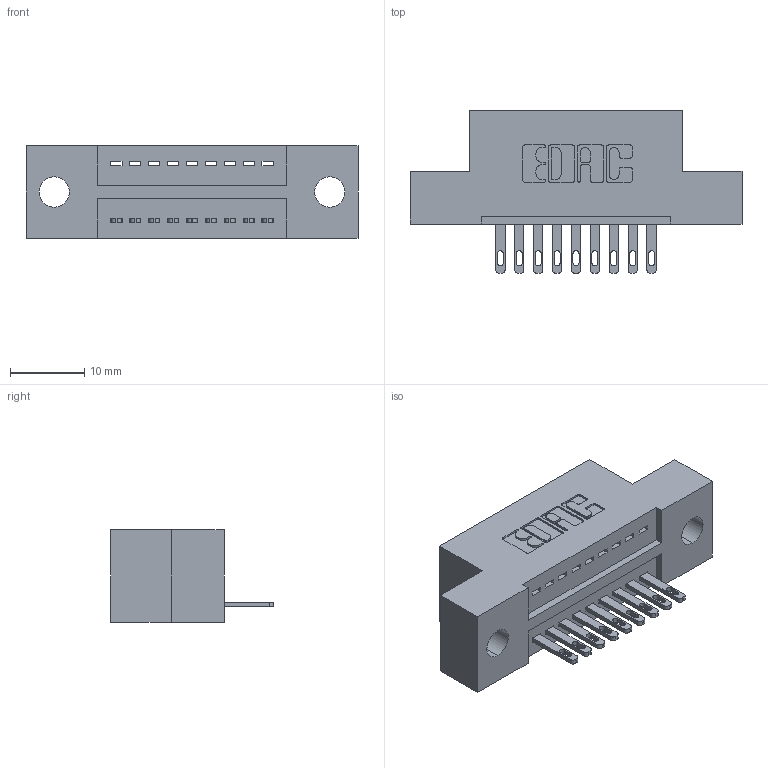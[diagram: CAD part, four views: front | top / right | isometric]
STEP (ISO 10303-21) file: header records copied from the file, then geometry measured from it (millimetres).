
FILE_DESCRIPTION (( 'STEP AP203' ), '1' );
FILE_NAME ('325-009-500-109.STEP', '2020-02-24T14:55:46', ( '' ), ( '' ), 'SwSTEP 2.0', 'SolidWorks 2016', '' );
FILE_SCHEMA (( 'CONFIG_CONTROL_DESIGN' ));
Length unit declared in the file: inch
Products named in the file (3): 325-292-001_325-293-100; 325-009-500-109; 325 Part_.160 TH
Assembly tree (10 placements, depth 2):
  325-009-500-109
    325 Part_.160 TH
    325-292-001_325-293-100  x9
Bounding box: 44.58 x 21.84 x 12.45 mm (x, y, z)
Volume: 5174.3 mm3; surface area: 5010 mm2
Topology: 10 solids, 10 shells, 600 faces, 1823 edges, 1214 vertices
Faces by surface type: plane 394, cylinder 206
Entity records: 9703 total; most frequent: CARTESIAN_POINT 1685, ORIENTED_EDGE 1630, DIRECTION 1489, EDGE_CURVE 815, LINE 683, VECTOR 683, VERTEX_POINT 542, AXIS2_PLACEMENT_3D 403
